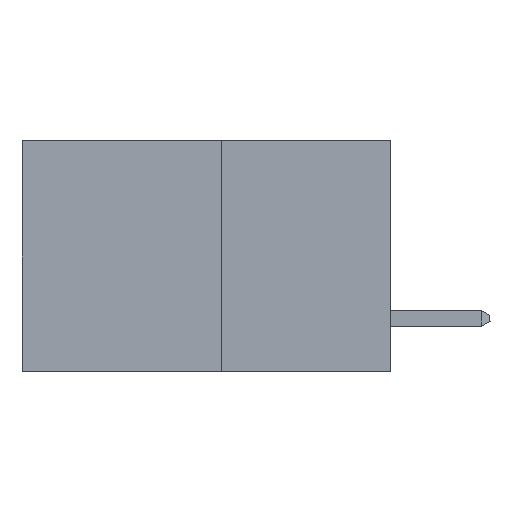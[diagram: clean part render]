
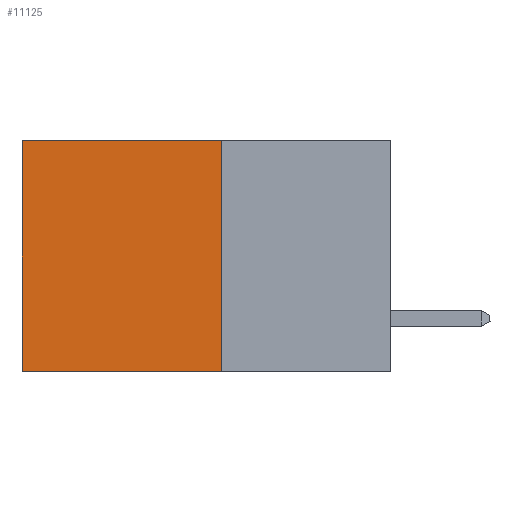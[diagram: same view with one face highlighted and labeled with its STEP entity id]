
A CAD part, left-side view. The second image highlights one B-rep face of the part: STEP entity #11125.
In plain terms, the highlighted planar face has unit normal (-1, 0, 0).
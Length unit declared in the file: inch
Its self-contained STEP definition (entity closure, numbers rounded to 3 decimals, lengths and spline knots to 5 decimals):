
#2164 = VERTEX_POINT ( 'NONE', #7847 ) ;
#3598 = LINE ( 'NONE', #15028, #24001 ) ;
#4608 = VERTEX_POINT ( 'NONE', #17758 ) ;
#4892 = FACE_OUTER_BOUND ( 'NONE', #23717, .T. ) ;
#5272 = CARTESIAN_POINT ( 'NONE',  ( 0.277, 0.27, -0.37 ) ) ;
#5460 = DIRECTION ( 'NONE',  ( 0., 0., -1. ) ) ;
#6693 = ORIENTED_EDGE ( 'NONE', *, *, #16921, .T. ) ;
#7739 = VECTOR ( 'NONE', #13796, 39.37008 ) ;
#7847 = CARTESIAN_POINT ( 'NONE',  ( 0.277, 0.59, 0. ) ) ;
#7946 = CARTESIAN_POINT ( 'NONE',  ( 0.277, 0.27, 0. ) ) ;
#8073 = LINE ( 'NONE', #9529, #22782 ) ;
#8711 = ORIENTED_EDGE ( 'NONE', *, *, #18207, .F. ) ;
#9529 = CARTESIAN_POINT ( 'NONE',  ( 0.277, 0.27, -0.37 ) ) ;
#9692 = VERTEX_POINT ( 'NONE', #17856 ) ;
#9993 = CARTESIAN_POINT ( 'NONE',  ( 0.277, 0.59, -0.37 ) ) ;
#11039 = DIRECTION ( 'NONE',  ( 0., 0., -1. ) ) ;
#11125 = ADVANCED_FACE ( 'NONE', ( #4892 ), #12897, .F. ) ;
#11475 = DIRECTION ( 'NONE',  ( 0., 1., 0. ) ) ;
#12897 = PLANE ( 'NONE',  #15773 ) ;
#13796 = DIRECTION ( 'NONE',  ( 0., 0., -1. ) ) ;
#14033 = EDGE_CURVE ( 'NONE', #2164, #20320, #23029, .T. ) ;
#15028 = CARTESIAN_POINT ( 'NONE',  ( 0.277, 0.27, -0.37 ) ) ;
#15773 = AXIS2_PLACEMENT_3D ( 'NONE', #5272, #22555, #11039 ) ;
#15858 = ORIENTED_EDGE ( 'NONE', *, *, #14033, .T. ) ;
#16921 = EDGE_CURVE ( 'NONE', #4608, #2164, #24075, .T. ) ;
#17612 = DIRECTION ( 'NONE',  ( 0., 1., 0. ) ) ;
#17758 = CARTESIAN_POINT ( 'NONE',  ( 0.277, 0.27, 0. ) ) ;
#17856 = CARTESIAN_POINT ( 'NONE',  ( 0.277, 0.27, -0.37 ) ) ;
#18207 = EDGE_CURVE ( 'NONE', #4608, #9692, #3598, .T. ) ;
#18240 = CARTESIAN_POINT ( 'NONE',  ( 0.277, 0.59, -0.37 ) ) ;
#18346 = ORIENTED_EDGE ( 'NONE', *, *, #24427, .F. ) ;
#18995 = VECTOR ( 'NONE', #17612, 39.37008 ) ;
#20320 = VERTEX_POINT ( 'NONE', #18240 ) ;
#22555 = DIRECTION ( 'NONE',  ( 1., 0., 0. ) ) ;
#22782 = VECTOR ( 'NONE', #11475, 39.37008 ) ;
#23029 = LINE ( 'NONE', #9993, #7739 ) ;
#23717 = EDGE_LOOP ( 'NONE', ( #15858, #18346, #8711, #6693 ) ) ;
#24001 = VECTOR ( 'NONE', #5460, 39.37008 ) ;
#24075 = LINE ( 'NONE', #7946, #18995 ) ;
#24427 = EDGE_CURVE ( 'NONE', #9692, #20320, #8073, .T. ) ;
